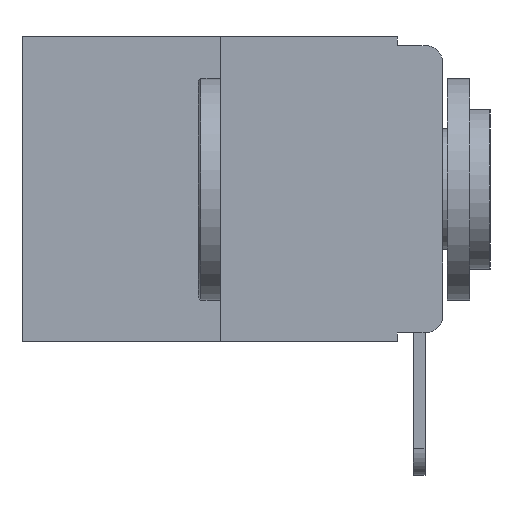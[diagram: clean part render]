
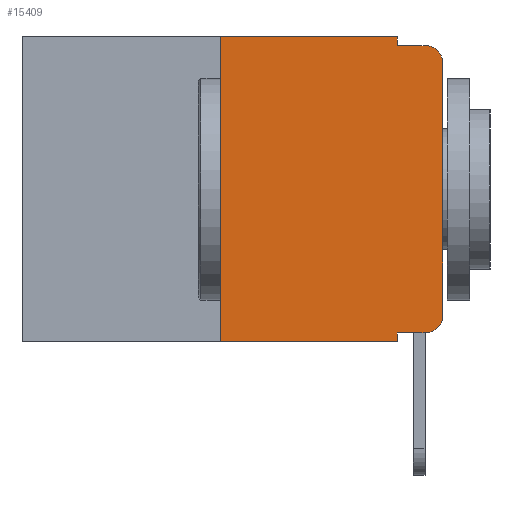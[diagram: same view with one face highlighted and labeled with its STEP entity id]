
A CAD part, left-side view. The second image highlights one B-rep face of the part: STEP entity #15409.
In plain terms, the highlighted planar face has unit normal (-1, 0, 0).
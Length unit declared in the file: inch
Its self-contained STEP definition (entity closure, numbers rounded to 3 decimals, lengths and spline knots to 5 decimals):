
#55 = ORIENTED_EDGE ( 'NONE', *, *, #2319, .F. ) ;
#388 = VECTOR ( 'NONE', #13280, 39.37008 ) ;
#400 = LINE ( 'NONE', #789, #5011 ) ;
#789 = CARTESIAN_POINT ( 'NONE',  ( 0., 0.473, -0.343 ) ) ;
#808 = LINE ( 'NONE', #14872, #9697 ) ;
#885 = VERTEX_POINT ( 'NONE', #12110 ) ;
#901 = ORIENTED_EDGE ( 'NONE', *, *, #9661, .T. ) ;
#1007 = CARTESIAN_POINT ( 'NONE',  ( 0., 0.473, 0. ) ) ;
#1159 = CARTESIAN_POINT ( 'NONE',  ( 0., 0.25, -0.343 ) ) ;
#1429 = EDGE_CURVE ( 'NONE', #8536, #13656, #15131, .T. ) ;
#1502 = ORIENTED_EDGE ( 'NONE', *, *, #6577, .T. ) ;
#1578 = VERTEX_POINT ( 'NONE', #6317 ) ;
#1585 = EDGE_CURVE ( 'NONE', #885, #8458, #808, .T. ) ;
#1904 = DIRECTION ( 'NONE',  ( -1., 0., 0. ) ) ;
#2045 = DIRECTION ( 'NONE',  ( 0., -1., 0. ) ) ;
#2068 = DIRECTION ( 'NONE',  ( 0., 0., -1. ) ) ;
#2096 = PLANE ( 'NONE',  #6509 ) ;
#2319 = EDGE_CURVE ( 'NONE', #885, #11934, #10267, .T. ) ;
#2325 = ORIENTED_EDGE ( 'NONE', *, *, #1429, .F. ) ;
#2366 = EDGE_CURVE ( 'NONE', #7832, #11934, #400, .T. ) ;
#2633 = CARTESIAN_POINT ( 'NONE',  ( 0., 0.02, -0.01 ) ) ;
#2931 = VECTOR ( 'NONE', #8062, 39.37008 ) ;
#3090 = CARTESIAN_POINT ( 'NONE',  ( 0., 0., -0.03 ) ) ;
#3126 = DIRECTION ( 'NONE',  ( 0., -1., 0. ) ) ;
#3244 = EDGE_CURVE ( 'NONE', #7832, #12701, #5410, .T. ) ;
#3723 = CIRCLE ( 'NONE', #10565, 0.02 ) ;
#5011 = VECTOR ( 'NONE', #2045, 39.37008 ) ;
#5238 = VECTOR ( 'NONE', #3126, 39.37008 ) ;
#5410 = LINE ( 'NONE', #9838, #12972 ) ;
#5685 = EDGE_LOOP ( 'NONE', ( #901, #7274, #2325, #12697, #7551, #5874, #12560, #55, #16011, #1502 ) ) ;
#5874 = ORIENTED_EDGE ( 'NONE', *, *, #3244, .F. ) ;
#6201 = AXIS2_PLACEMENT_3D ( 'NONE', #15962, #14621, #14667 ) ;
#6317 = CARTESIAN_POINT ( 'NONE',  ( 0., 0.051, 0. ) ) ;
#6509 = AXIS2_PLACEMENT_3D ( 'NONE', #8014, #10681, #15595 ) ;
#6577 = EDGE_CURVE ( 'NONE', #8458, #6648, #3723, .T. ) ;
#6648 = VERTEX_POINT ( 'NONE', #14837 ) ;
#7274 = ORIENTED_EDGE ( 'NONE', *, *, #15986, .T. ) ;
#7409 = DIRECTION ( 'NONE',  ( 0., 0., 1. ) ) ;
#7550 = EDGE_CURVE ( 'NONE', #1578, #8536, #13746, .T. ) ;
#7551 = ORIENTED_EDGE ( 'NONE', *, *, #15197, .F. ) ;
#7832 = VERTEX_POINT ( 'NONE', #1159 ) ;
#8014 = CARTESIAN_POINT ( 'NONE',  ( 0., 0.473, 0. ) ) ;
#8021 = CARTESIAN_POINT ( 'NONE',  ( 0., 0.051, -0.01 ) ) ;
#8062 = DIRECTION ( 'NONE',  ( 0., 0., -1. ) ) ;
#8141 = VECTOR ( 'NONE', #9438, 39.37008 ) ;
#8458 = VERTEX_POINT ( 'NONE', #11201 ) ;
#8536 = VERTEX_POINT ( 'NONE', #13671 ) ;
#9438 = DIRECTION ( 'NONE',  ( 0., 0., -1. ) ) ;
#9661 = EDGE_CURVE ( 'NONE', #6648, #11588, #11219, .T. ) ;
#9697 = VECTOR ( 'NONE', #15028, 39.37008 ) ;
#9838 = CARTESIAN_POINT ( 'NONE',  ( 0., 0.25, 0. ) ) ;
#9951 = DIRECTION ( 'NONE',  ( 0., 0., 1. ) ) ;
#10092 = CARTESIAN_POINT ( 'NONE',  ( 0., 0.051, -0.343 ) ) ;
#10267 = LINE ( 'NONE', #14356, #8141 ) ;
#10565 = AXIS2_PLACEMENT_3D ( 'NONE', #11852, #1904, #2068 ) ;
#10681 = DIRECTION ( 'NONE',  ( 1., 0., 0. ) ) ;
#11201 = CARTESIAN_POINT ( 'NONE',  ( 0., 0.02, -0.333 ) ) ;
#11219 = LINE ( 'NONE', #16014, #15066 ) ;
#11588 = VERTEX_POINT ( 'NONE', #3090 ) ;
#11654 = CARTESIAN_POINT ( 'NONE',  ( 0., 0.051, 0. ) ) ;
#11699 = CARTESIAN_POINT ( 'NONE',  ( 0., 0.25, 0. ) ) ;
#11852 = CARTESIAN_POINT ( 'NONE',  ( 0., 0.02, -0.313 ) ) ;
#11934 = VERTEX_POINT ( 'NONE', #10092 ) ;
#12110 = CARTESIAN_POINT ( 'NONE',  ( 0., 0.051, -0.333 ) ) ;
#12560 = ORIENTED_EDGE ( 'NONE', *, *, #2366, .T. ) ;
#12697 = ORIENTED_EDGE ( 'NONE', *, *, #7550, .F. ) ;
#12701 = VERTEX_POINT ( 'NONE', #11699 ) ;
#12972 = VECTOR ( 'NONE', #9951, 39.37008 ) ;
#13280 = DIRECTION ( 'NONE',  ( 0., -1., 0. ) ) ;
#13547 = LINE ( 'NONE', #1007, #388 ) ;
#13656 = VERTEX_POINT ( 'NONE', #2633 ) ;
#13671 = CARTESIAN_POINT ( 'NONE',  ( 0., 0.051, -0.01 ) ) ;
#13746 = LINE ( 'NONE', #11654, #2931 ) ;
#13983 = CIRCLE ( 'NONE', #6201, 0.02 ) ;
#14114 = FACE_OUTER_BOUND ( 'NONE', #5685, .T. ) ;
#14356 = CARTESIAN_POINT ( 'NONE',  ( 0., 0.051, 0. ) ) ;
#14621 = DIRECTION ( 'NONE',  ( -1., 0., 0. ) ) ;
#14667 = DIRECTION ( 'NONE',  ( 0., 0., -1. ) ) ;
#14837 = CARTESIAN_POINT ( 'NONE',  ( 0., 0., -0.313 ) ) ;
#14872 = CARTESIAN_POINT ( 'NONE',  ( 0., 0.051, -0.333 ) ) ;
#15028 = DIRECTION ( 'NONE',  ( 0., -1., 0. ) ) ;
#15066 = VECTOR ( 'NONE', #7409, 39.37008 ) ;
#15131 = LINE ( 'NONE', #8021, #5238 ) ;
#15197 = EDGE_CURVE ( 'NONE', #12701, #1578, #13547, .T. ) ;
#15409 = ADVANCED_FACE ( 'NONE', ( #14114 ), #2096, .F. ) ;
#15595 = DIRECTION ( 'NONE',  ( 0., 0., -1. ) ) ;
#15962 = CARTESIAN_POINT ( 'NONE',  ( 0., 0.02, -0.03 ) ) ;
#15986 = EDGE_CURVE ( 'NONE', #11588, #13656, #13983, .T. ) ;
#16011 = ORIENTED_EDGE ( 'NONE', *, *, #1585, .T. ) ;
#16014 = CARTESIAN_POINT ( 'NONE',  ( 0., 0., 0. ) ) ;
